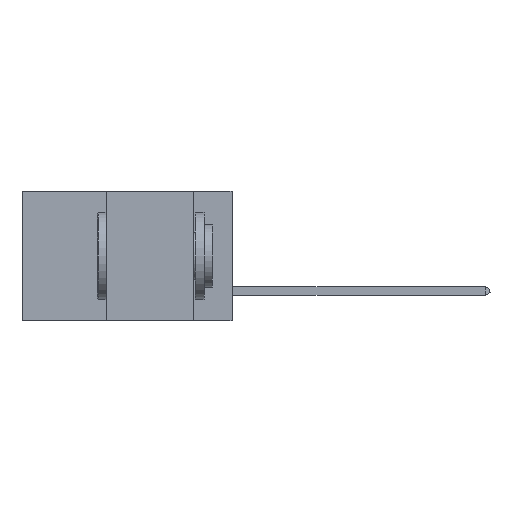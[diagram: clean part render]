
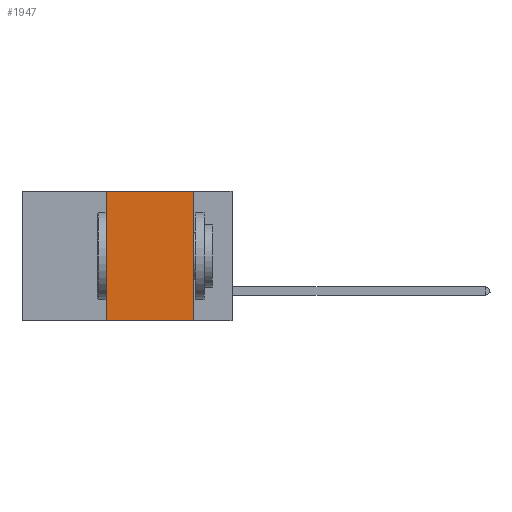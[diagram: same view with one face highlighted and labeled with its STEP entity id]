
A CAD part, left-side view. The second image highlights one B-rep face of the part: STEP entity #1947.
In plain terms, the highlighted planar face has unit normal (-1, 0, 0).
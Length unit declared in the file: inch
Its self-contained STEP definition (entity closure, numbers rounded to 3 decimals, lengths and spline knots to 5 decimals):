
#1947 = ADVANCED_FACE ( 'NONE', ( #10302 ), #5030, .F. ) ;
#2784 = CARTESIAN_POINT ( 'NONE',  ( 0., 0.36, -0.37 ) ) ;
#3040 = CARTESIAN_POINT ( 'NONE',  ( 0., 0.11, 0. ) ) ;
#3330 = DIRECTION ( 'NONE',  ( 0., -1., 0. ) ) ;
#5030 = PLANE ( 'NONE',  #22086 ) ;
#5369 = ORIENTED_EDGE ( 'NONE', *, *, #13246, .F. ) ;
#7399 = DIRECTION ( 'NONE',  ( 1., 0., 0. ) ) ;
#7653 = VERTEX_POINT ( 'NONE', #11181 ) ;
#8627 = VECTOR ( 'NONE', #25727, 39.37008 ) ;
#8691 = EDGE_CURVE ( 'NONE', #28685, #15811, #26873, .T. ) ;
#8769 = VECTOR ( 'NONE', #9949, 39.37008 ) ;
#9949 = DIRECTION ( 'NONE',  ( 0., -1., 0. ) ) ;
#10302 = FACE_OUTER_BOUND ( 'NONE', #26899, .T. ) ;
#11181 = CARTESIAN_POINT ( 'NONE',  ( 0., 0.11, -0.37 ) ) ;
#11946 = EDGE_CURVE ( 'NONE', #20202, #7653, #23596, .T. ) ;
#12421 = LINE ( 'NONE', #3040, #17985 ) ;
#13246 = EDGE_CURVE ( 'NONE', #15811, #7653, #12421, .T. ) ;
#15811 = VERTEX_POINT ( 'NONE', #29418 ) ;
#16846 = CARTESIAN_POINT ( 'NONE',  ( 0., 0.6, -0.37 ) ) ;
#17985 = VECTOR ( 'NONE', #19544, 39.37008 ) ;
#19044 = ORIENTED_EDGE ( 'NONE', *, *, #11946, .T. ) ;
#19086 = CARTESIAN_POINT ( 'NONE',  ( 0., 0.6, 0. ) ) ;
#19544 = DIRECTION ( 'NONE',  ( 0., 0., -1. ) ) ;
#20202 = VERTEX_POINT ( 'NONE', #2784 ) ;
#20787 = EDGE_CURVE ( 'NONE', #20202, #28685, #26366, .T. ) ;
#20984 = CARTESIAN_POINT ( 'NONE',  ( 0., 0.36, 0. ) ) ;
#22086 = AXIS2_PLACEMENT_3D ( 'NONE', #26065, #7399, #26168 ) ;
#23596 = LINE ( 'NONE', #16846, #27651 ) ;
#23858 = CARTESIAN_POINT ( 'NONE',  ( 0., 0.36, 0. ) ) ;
#24292 = ORIENTED_EDGE ( 'NONE', *, *, #20787, .F. ) ;
#24890 = ORIENTED_EDGE ( 'NONE', *, *, #8691, .F. ) ;
#25727 = DIRECTION ( 'NONE',  ( 0., 0., 1. ) ) ;
#26065 = CARTESIAN_POINT ( 'NONE',  ( 0., 0.6, 0. ) ) ;
#26168 = DIRECTION ( 'NONE',  ( 0., 0., -1. ) ) ;
#26366 = LINE ( 'NONE', #20984, #8627 ) ;
#26873 = LINE ( 'NONE', #19086, #8769 ) ;
#26899 = EDGE_LOOP ( 'NONE', ( #5369, #24890, #24292, #19044 ) ) ;
#27651 = VECTOR ( 'NONE', #3330, 39.37008 ) ;
#28685 = VERTEX_POINT ( 'NONE', #23858 ) ;
#29418 = CARTESIAN_POINT ( 'NONE',  ( 0., 0.11, 0. ) ) ;
